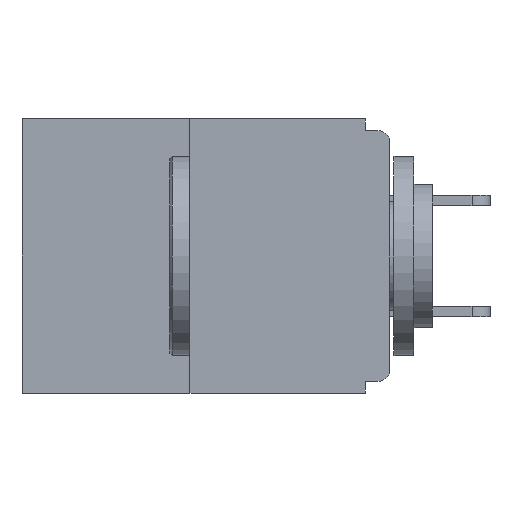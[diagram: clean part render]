
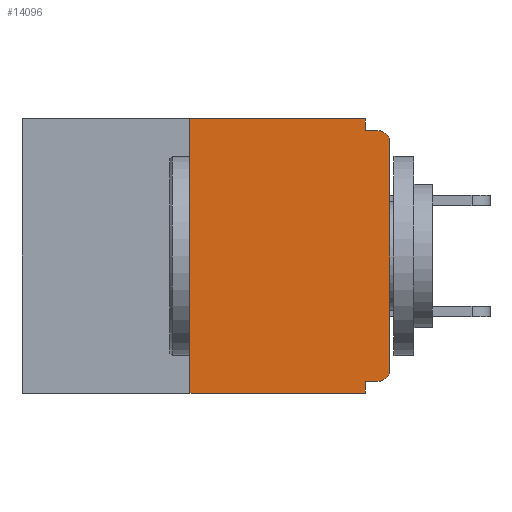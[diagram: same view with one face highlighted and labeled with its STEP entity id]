
A CAD part, left-side view. The second image highlights one B-rep face of the part: STEP entity #14096.
In plain terms, the highlighted planar face has unit normal (-1, 0, 0).
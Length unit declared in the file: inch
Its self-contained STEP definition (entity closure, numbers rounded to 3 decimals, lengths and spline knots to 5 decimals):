
#200 = AXIS2_PLACEMENT_3D ( 'NONE', #4962, #18213, #21919 ) ;
#429 = ORIENTED_EDGE ( 'NONE', *, *, #8684, .T. ) ;
#569 = VECTOR ( 'NONE', #23364, 39.37008 ) ;
#644 = CARTESIAN_POINT ( 'NONE',  ( 0., 0.46, 0. ) ) ;
#910 = EDGE_CURVE ( 'NONE', #8779, #18372, #22051, .T. ) ;
#1003 = CARTESIAN_POINT ( 'NONE',  ( 0., 0.25, -0.343 ) ) ;
#1133 = CARTESIAN_POINT ( 'NONE',  ( 0., 0.031, -0.015 ) ) ;
#1558 = VERTEX_POINT ( 'NONE', #14828 ) ;
#1944 = CARTESIAN_POINT ( 'NONE',  ( 0., 0., 0. ) ) ;
#2402 = DIRECTION ( 'NONE',  ( 0., 1., 0. ) ) ;
#2957 = ORIENTED_EDGE ( 'NONE', *, *, #20868, .F. ) ;
#3702 = CARTESIAN_POINT ( 'NONE',  ( 0., 0.031, -0.328 ) ) ;
#3991 = EDGE_CURVE ( 'NONE', #8779, #19881, #6571, .T. ) ;
#4086 = CARTESIAN_POINT ( 'NONE',  ( 0., 0., -0.313 ) ) ;
#4309 = VECTOR ( 'NONE', #14526, 39.37008 ) ;
#4962 = CARTESIAN_POINT ( 'NONE',  ( 0., 0.015, -0.03 ) ) ;
#4965 = AXIS2_PLACEMENT_3D ( 'NONE', #644, #21371, #10132 ) ;
#5134 = DIRECTION ( 'NONE',  ( 0., 0., 1. ) ) ;
#5207 = ORIENTED_EDGE ( 'NONE', *, *, #16014, .F. ) ;
#5242 = VECTOR ( 'NONE', #2402, 39.37008 ) ;
#6384 = ORIENTED_EDGE ( 'NONE', *, *, #22681, .F. ) ;
#6426 = VECTOR ( 'NONE', #10370, 39.37008 ) ;
#6571 = CIRCLE ( 'NONE', #14593, 0.015 ) ;
#7063 = CARTESIAN_POINT ( 'NONE',  ( 0., 0.015, -0.015 ) ) ;
#7090 = ORIENTED_EDGE ( 'NONE', *, *, #11852, .F. ) ;
#7116 = DIRECTION ( 'NONE',  ( -1., 0., 0. ) ) ;
#7292 = ORIENTED_EDGE ( 'NONE', *, *, #20782, .T. ) ;
#7558 = CIRCLE ( 'NONE', #200, 0.015 ) ;
#7584 = DIRECTION ( 'NONE',  ( 0., 0., -1. ) ) ;
#7634 = LINE ( 'NONE', #23216, #6426 ) ;
#8293 = CARTESIAN_POINT ( 'NONE',  ( 0., 0., -0.015 ) ) ;
#8684 = EDGE_CURVE ( 'NONE', #14884, #1558, #22412, .T. ) ;
#8703 = EDGE_LOOP ( 'NONE', ( #5207, #2957, #429, #7090, #17220, #10745, #12104, #7292, #13804, #6384 ) ) ;
#8779 = VERTEX_POINT ( 'NONE', #20217 ) ;
#10132 = DIRECTION ( 'NONE',  ( 0., 0., -1. ) ) ;
#10370 = DIRECTION ( 'NONE',  ( 0., -1., 0. ) ) ;
#10675 = VECTOR ( 'NONE', #7584, 39.37008 ) ;
#10745 = ORIENTED_EDGE ( 'NONE', *, *, #3991, .T. ) ;
#10865 = DIRECTION ( 'NONE',  ( 0., 0., -1. ) ) ;
#11852 = EDGE_CURVE ( 'NONE', #18372, #1558, #21078, .T. ) ;
#11953 = LINE ( 'NONE', #14765, #18170 ) ;
#12104 = ORIENTED_EDGE ( 'NONE', *, *, #13363, .T. ) ;
#12768 = CARTESIAN_POINT ( 'NONE',  ( 0., 0.015, -0.313 ) ) ;
#13363 = EDGE_CURVE ( 'NONE', #19881, #23606, #16282, .T. ) ;
#13684 = LINE ( 'NONE', #20837, #10675 ) ;
#13804 = ORIENTED_EDGE ( 'NONE', *, *, #19652, .F. ) ;
#14096 = ADVANCED_FACE ( 'NONE', ( #14501 ), #23200, .F. ) ;
#14501 = FACE_OUTER_BOUND ( 'NONE', #8703, .T. ) ;
#14526 = DIRECTION ( 'NONE',  ( 0., 0., -1. ) ) ;
#14593 = AXIS2_PLACEMENT_3D ( 'NONE', #12768, #7116, #10865 ) ;
#14747 = CARTESIAN_POINT ( 'NONE',  ( 0., 0., -0.328 ) ) ;
#14765 = CARTESIAN_POINT ( 'NONE',  ( 0., 0.25, 0. ) ) ;
#14828 = CARTESIAN_POINT ( 'NONE',  ( 0., 0.031, -0.343 ) ) ;
#14884 = VERTEX_POINT ( 'NONE', #1003 ) ;
#15099 = DIRECTION ( 'NONE',  ( 0., 0., 1. ) ) ;
#15644 = VECTOR ( 'NONE', #23609, 39.37008 ) ;
#15859 = VERTEX_POINT ( 'NONE', #16068 ) ;
#16014 = EDGE_CURVE ( 'NONE', #15859, #16614, #7634, .T. ) ;
#16068 = CARTESIAN_POINT ( 'NONE',  ( 0., 0.25, 0. ) ) ;
#16160 = CARTESIAN_POINT ( 'NONE',  ( 0., 0., -0.03 ) ) ;
#16282 = LINE ( 'NONE', #1944, #17804 ) ;
#16432 = LINE ( 'NONE', #8293, #569 ) ;
#16614 = VERTEX_POINT ( 'NONE', #18007 ) ;
#17220 = ORIENTED_EDGE ( 'NONE', *, *, #910, .F. ) ;
#17804 = VECTOR ( 'NONE', #15099, 39.37008 ) ;
#18007 = CARTESIAN_POINT ( 'NONE',  ( 0., 0.031, 0. ) ) ;
#18122 = CARTESIAN_POINT ( 'NONE',  ( 0., 0.46, -0.343 ) ) ;
#18170 = VECTOR ( 'NONE', #5134, 39.37008 ) ;
#18209 = VERTEX_POINT ( 'NONE', #7063 ) ;
#18213 = DIRECTION ( 'NONE',  ( -1., 0., 0. ) ) ;
#18316 = CARTESIAN_POINT ( 'NONE',  ( 0., 0.031, -0.343 ) ) ;
#18372 = VERTEX_POINT ( 'NONE', #3702 ) ;
#19652 = EDGE_CURVE ( 'NONE', #23460, #18209, #16432, .T. ) ;
#19881 = VERTEX_POINT ( 'NONE', #4086 ) ;
#20217 = CARTESIAN_POINT ( 'NONE',  ( 0., 0.015, -0.328 ) ) ;
#20782 = EDGE_CURVE ( 'NONE', #23606, #18209, #7558, .T. ) ;
#20837 = CARTESIAN_POINT ( 'NONE',  ( 0., 0.031, 0. ) ) ;
#20868 = EDGE_CURVE ( 'NONE', #14884, #15859, #11953, .T. ) ;
#21078 = LINE ( 'NONE', #18316, #4309 ) ;
#21371 = DIRECTION ( 'NONE',  ( 1., 0., 0. ) ) ;
#21919 = DIRECTION ( 'NONE',  ( 0., 0., -1. ) ) ;
#22051 = LINE ( 'NONE', #14747, #5242 ) ;
#22412 = LINE ( 'NONE', #18122, #15644 ) ;
#22681 = EDGE_CURVE ( 'NONE', #16614, #23460, #13684, .T. ) ;
#23200 = PLANE ( 'NONE',  #4965 ) ;
#23216 = CARTESIAN_POINT ( 'NONE',  ( 0., 0.46, 0. ) ) ;
#23364 = DIRECTION ( 'NONE',  ( 0., -1., 0. ) ) ;
#23460 = VERTEX_POINT ( 'NONE', #1133 ) ;
#23606 = VERTEX_POINT ( 'NONE', #16160 ) ;
#23609 = DIRECTION ( 'NONE',  ( 0., -1., 0. ) ) ;
